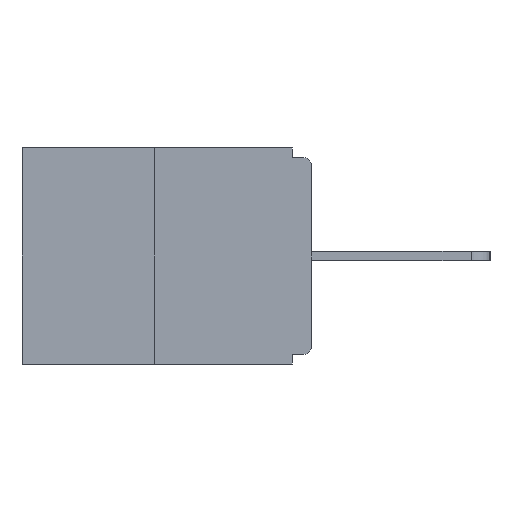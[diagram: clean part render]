
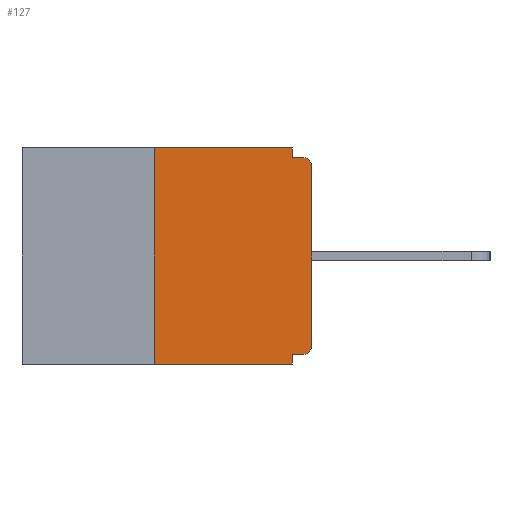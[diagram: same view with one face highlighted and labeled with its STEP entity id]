
A CAD part, left-side view. The second image highlights one B-rep face of the part: STEP entity #127.
In plain terms, the highlighted planar face has unit normal (-1, 0, 0).
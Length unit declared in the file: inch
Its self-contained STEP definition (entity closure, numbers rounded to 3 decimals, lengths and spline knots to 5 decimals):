
#32 = VECTOR ( 'NONE', #5198, 39.37008 ) ;
#127 = ADVANCED_FACE ( 'NONE', ( #909 ), #18893, .F. ) ;
#171 = CARTESIAN_POINT ( 'NONE',  ( 0., 0., -0.03 ) ) ;
#345 = LINE ( 'NONE', #13475, #8469 ) ;
#482 = LINE ( 'NONE', #17068, #32 ) ;
#667 = ORIENTED_EDGE ( 'NONE', *, *, #18041, .F. ) ;
#806 = CARTESIAN_POINT ( 'NONE',  ( 0., 0.031, -0.015 ) ) ;
#909 = FACE_OUTER_BOUND ( 'NONE', #2744, .T. ) ;
#1477 = CARTESIAN_POINT ( 'NONE',  ( 0., 0.031, -0.328 ) ) ;
#1859 = LINE ( 'NONE', #15424, #20403 ) ;
#1920 = DIRECTION ( 'NONE',  ( 0., 0., -1. ) ) ;
#2303 = DIRECTION ( 'NONE',  ( 0., -1., 0. ) ) ;
#2743 = EDGE_CURVE ( 'NONE', #3201, #4000, #4884, .T. ) ;
#2744 = EDGE_LOOP ( 'NONE', ( #667, #8135, #17493, #20573, #14748, #15808, #10166, #5796, #10278, #13008 ) ) ;
#2857 = DIRECTION ( 'NONE',  ( -1., 0., 0. ) ) ;
#2904 = VERTEX_POINT ( 'NONE', #171 ) ;
#3051 = VECTOR ( 'NONE', #11141, 39.37008 ) ;
#3201 = VERTEX_POINT ( 'NONE', #6596 ) ;
#3782 = VECTOR ( 'NONE', #7008, 39.37008 ) ;
#3793 = EDGE_CURVE ( 'NONE', #7305, #7601, #1859, .T. ) ;
#4000 = VERTEX_POINT ( 'NONE', #11512 ) ;
#4471 = CARTESIAN_POINT ( 'NONE',  ( 0., 0.015, -0.313 ) ) ;
#4696 = CARTESIAN_POINT ( 'NONE',  ( 0., 0.015, -0.015 ) ) ;
#4884 = LINE ( 'NONE', #11472, #3051 ) ;
#4938 = LINE ( 'NONE', #11528, #19012 ) ;
#5198 = DIRECTION ( 'NONE',  ( 0., -1., 0. ) ) ;
#5796 = ORIENTED_EDGE ( 'NONE', *, *, #16250, .T. ) ;
#6596 = CARTESIAN_POINT ( 'NONE',  ( 0., 0.25, -0.343 ) ) ;
#7008 = DIRECTION ( 'NONE',  ( 0., 0., 1. ) ) ;
#7044 = CARTESIAN_POINT ( 'NONE',  ( 0., 0.015, -0.328 ) ) ;
#7129 = CARTESIAN_POINT ( 'NONE',  ( 0., 0., -0.015 ) ) ;
#7305 = VERTEX_POINT ( 'NONE', #19450 ) ;
#7329 = LINE ( 'NONE', #13704, #3782 ) ;
#7601 = VERTEX_POINT ( 'NONE', #806 ) ;
#7632 = VECTOR ( 'NONE', #2303, 39.37008 ) ;
#7987 = DIRECTION ( 'NONE',  ( 0., 1., 0. ) ) ;
#7989 = VECTOR ( 'NONE', #14677, 39.37008 ) ;
#8055 = EDGE_CURVE ( 'NONE', #13139, #2904, #7329, .T. ) ;
#8098 = LINE ( 'NONE', #18211, #7989 ) ;
#8135 = ORIENTED_EDGE ( 'NONE', *, *, #14904, .F. ) ;
#8220 = VERTEX_POINT ( 'NONE', #15747 ) ;
#8371 = AXIS2_PLACEMENT_3D ( 'NONE', #4471, #2857, #10635 ) ;
#8469 = VECTOR ( 'NONE', #11840, 39.37008 ) ;
#9095 = CARTESIAN_POINT ( 'NONE',  ( 0., 0., -0.313 ) ) ;
#9374 = EDGE_CURVE ( 'NONE', #7601, #16233, #15326, .T. ) ;
#9488 = CIRCLE ( 'NONE', #12223, 0.015 ) ;
#9609 = EDGE_CURVE ( 'NONE', #14101, #19138, #4938, .T. ) ;
#9676 = EDGE_CURVE ( 'NONE', #19138, #4000, #8098, .T. ) ;
#9785 = DIRECTION ( 'NONE',  ( -1., 0., 0. ) ) ;
#9998 = CARTESIAN_POINT ( 'NONE',  ( 0., 0.46, 0. ) ) ;
#10166 = ORIENTED_EDGE ( 'NONE', *, *, #8055, .T. ) ;
#10278 = ORIENTED_EDGE ( 'NONE', *, *, #9374, .F. ) ;
#10288 = EDGE_CURVE ( 'NONE', #14101, #13139, #17643, .T. ) ;
#10524 = DIRECTION ( 'NONE',  ( 0., 0., -1. ) ) ;
#10635 = DIRECTION ( 'NONE',  ( 0., 0., -1. ) ) ;
#11141 = DIRECTION ( 'NONE',  ( 0., -1., 0. ) ) ;
#11472 = CARTESIAN_POINT ( 'NONE',  ( 0., 0.46, -0.343 ) ) ;
#11512 = CARTESIAN_POINT ( 'NONE',  ( 0., 0.031, -0.343 ) ) ;
#11528 = CARTESIAN_POINT ( 'NONE',  ( 0., 0., -0.328 ) ) ;
#11840 = DIRECTION ( 'NONE',  ( 0., 0., 1. ) ) ;
#12223 = AXIS2_PLACEMENT_3D ( 'NONE', #13010, #9785, #10524 ) ;
#13008 = ORIENTED_EDGE ( 'NONE', *, *, #3793, .F. ) ;
#13010 = CARTESIAN_POINT ( 'NONE',  ( 0., 0.015, -0.03 ) ) ;
#13139 = VERTEX_POINT ( 'NONE', #9095 ) ;
#13222 = DIRECTION ( 'NONE',  ( 1., 0., 0. ) ) ;
#13475 = CARTESIAN_POINT ( 'NONE',  ( 0., 0.25, 0. ) ) ;
#13704 = CARTESIAN_POINT ( 'NONE',  ( 0., 0., 0. ) ) ;
#14101 = VERTEX_POINT ( 'NONE', #7044 ) ;
#14677 = DIRECTION ( 'NONE',  ( 0., 0., -1. ) ) ;
#14748 = ORIENTED_EDGE ( 'NONE', *, *, #9609, .F. ) ;
#14904 = EDGE_CURVE ( 'NONE', #3201, #8220, #345, .T. ) ;
#15326 = LINE ( 'NONE', #7129, #7632 ) ;
#15424 = CARTESIAN_POINT ( 'NONE',  ( 0., 0.031, 0. ) ) ;
#15747 = CARTESIAN_POINT ( 'NONE',  ( 0., 0.25, 0. ) ) ;
#15808 = ORIENTED_EDGE ( 'NONE', *, *, #10288, .T. ) ;
#16233 = VERTEX_POINT ( 'NONE', #4696 ) ;
#16250 = EDGE_CURVE ( 'NONE', #2904, #16233, #9488, .T. ) ;
#16614 = DIRECTION ( 'NONE',  ( 0., 0., -1. ) ) ;
#17068 = CARTESIAN_POINT ( 'NONE',  ( 0., 0.46, 0. ) ) ;
#17493 = ORIENTED_EDGE ( 'NONE', *, *, #2743, .T. ) ;
#17643 = CIRCLE ( 'NONE', #8371, 0.015 ) ;
#18041 = EDGE_CURVE ( 'NONE', #8220, #7305, #482, .T. ) ;
#18211 = CARTESIAN_POINT ( 'NONE',  ( 0., 0.031, -0.343 ) ) ;
#18893 = PLANE ( 'NONE',  #20842 ) ;
#19012 = VECTOR ( 'NONE', #7987, 39.37008 ) ;
#19138 = VERTEX_POINT ( 'NONE', #1477 ) ;
#19450 = CARTESIAN_POINT ( 'NONE',  ( 0., 0.031, 0. ) ) ;
#20403 = VECTOR ( 'NONE', #16614, 39.37008 ) ;
#20573 = ORIENTED_EDGE ( 'NONE', *, *, #9676, .F. ) ;
#20842 = AXIS2_PLACEMENT_3D ( 'NONE', #9998, #13222, #1920 ) ;
